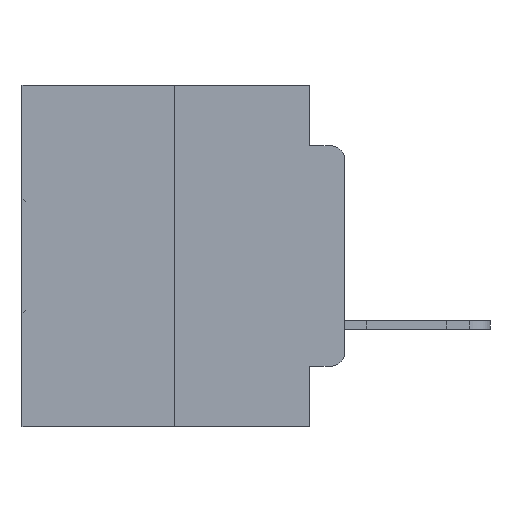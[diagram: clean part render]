
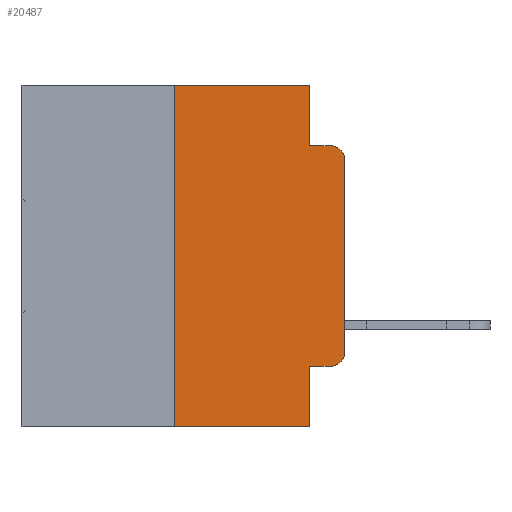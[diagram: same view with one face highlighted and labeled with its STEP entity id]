
A CAD part, left-side view. The second image highlights one B-rep face of the part: STEP entity #20487.
In plain terms, the highlighted planar face has unit normal (-1, 0, 0).
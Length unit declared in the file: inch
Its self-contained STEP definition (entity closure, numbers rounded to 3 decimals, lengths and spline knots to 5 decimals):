
#351 = VERTEX_POINT ( 'NONE', #5913 ) ;
#405 = VECTOR ( 'NONE', #18775, 39.37008 ) ;
#1139 = ORIENTED_EDGE ( 'NONE', *, *, #13608, .T. ) ;
#1945 = FACE_OUTER_BOUND ( 'NONE', #10490, .T. ) ;
#2028 = VECTOR ( 'NONE', #28562, 39.37008 ) ;
#2486 = LINE ( 'NONE', #10339, #12302 ) ;
#2933 = VERTEX_POINT ( 'NONE', #3479 ) ;
#3251 = VERTEX_POINT ( 'NONE', #19791 ) ;
#3339 = VECTOR ( 'NONE', #30224, 39.37008 ) ;
#3390 = VECTOR ( 'NONE', #20438, 39.37008 ) ;
#3479 = CARTESIAN_POINT ( 'NONE',  ( 0., 0.02, -0.0885 ) ) ;
#4576 = CARTESIAN_POINT ( 'NONE',  ( 0., 0., -0.3915 ) ) ;
#4650 = VERTEX_POINT ( 'NONE', #11251 ) ;
#5029 = DIRECTION ( 'NONE',  ( 1., 0., 0. ) ) ;
#5317 = AXIS2_PLACEMENT_3D ( 'NONE', #16862, #5029, #24354 ) ;
#5726 = ORIENTED_EDGE ( 'NONE', *, *, #31351, .T. ) ;
#5913 = CARTESIAN_POINT ( 'NONE',  ( 0., 0.25, -0.5 ) ) ;
#6045 = CARTESIAN_POINT ( 'NONE',  ( 0., 0.02, -0.1085 ) ) ;
#6817 = VECTOR ( 'NONE', #27521, 39.37008 ) ;
#6858 = CARTESIAN_POINT ( 'NONE',  ( 0., 0.051, -0.4115 ) ) ;
#6984 = DIRECTION ( 'NONE',  ( 0., 0., -1. ) ) ;
#7262 = CIRCLE ( 'NONE', #25867, 0.02 ) ;
#7264 = PLANE ( 'NONE',  #5317 ) ;
#8632 = CARTESIAN_POINT ( 'NONE',  ( 0., 0.473, 0. ) ) ;
#8911 = VECTOR ( 'NONE', #29484, 39.37008 ) ;
#9176 = ORIENTED_EDGE ( 'NONE', *, *, #18207, .F. ) ;
#9423 = CARTESIAN_POINT ( 'NONE',  ( 0., 0.051, 0. ) ) ;
#9775 = LINE ( 'NONE', #11331, #3339 ) ;
#9825 = LINE ( 'NONE', #27527, #3390 ) ;
#10070 = EDGE_CURVE ( 'NONE', #3251, #2933, #11827, .T. ) ;
#10143 = DIRECTION ( 'NONE',  ( 0., 0., -1. ) ) ;
#10339 = CARTESIAN_POINT ( 'NONE',  ( 0., 0.473, -0.5 ) ) ;
#10490 = EDGE_LOOP ( 'NONE', ( #5726, #25761, #30400, #30440, #9176, #28096, #1139, #11861, #22275, #29266 ) ) ;
#10564 = DIRECTION ( 'NONE',  ( 0., -1., 0. ) ) ;
#11251 = CARTESIAN_POINT ( 'NONE',  ( 0., 0.02, -0.4115 ) ) ;
#11331 = CARTESIAN_POINT ( 'NONE',  ( 0., 0.051, 0. ) ) ;
#11447 = EDGE_CURVE ( 'NONE', #21841, #3251, #9775, .T. ) ;
#11827 = LINE ( 'NONE', #21845, #405 ) ;
#11861 = ORIENTED_EDGE ( 'NONE', *, *, #20864, .F. ) ;
#12302 = VECTOR ( 'NONE', #10564, 39.37008 ) ;
#12610 = CARTESIAN_POINT ( 'NONE',  ( 0., 0.25, 0. ) ) ;
#12850 = CARTESIAN_POINT ( 'NONE',  ( 0., 0., 0. ) ) ;
#12901 = EDGE_CURVE ( 'NONE', #24994, #4650, #30842, .T. ) ;
#13608 = EDGE_CURVE ( 'NONE', #351, #26804, #2486, .T. ) ;
#13958 = DIRECTION ( 'NONE',  ( -1., 0., 0. ) ) ;
#15592 = DIRECTION ( 'NONE',  ( 0., 0., 1. ) ) ;
#16032 = VERTEX_POINT ( 'NONE', #23513 ) ;
#16079 = VERTEX_POINT ( 'NONE', #23188 ) ;
#16862 = CARTESIAN_POINT ( 'NONE',  ( 0., 0.473, 0. ) ) ;
#17411 = DIRECTION ( 'NONE',  ( -1., 0., 0. ) ) ;
#17823 = EDGE_CURVE ( 'NONE', #16032, #2933, #18289, .T. ) ;
#18207 = EDGE_CURVE ( 'NONE', #16079, #21841, #29977, .T. ) ;
#18289 = CIRCLE ( 'NONE', #25329, 0.02 ) ;
#18775 = DIRECTION ( 'NONE',  ( 0., -1., 0. ) ) ;
#19086 = VECTOR ( 'NONE', #15592, 39.37008 ) ;
#19791 = CARTESIAN_POINT ( 'NONE',  ( 0., 0.051, -0.0885 ) ) ;
#20438 = DIRECTION ( 'NONE',  ( 0., 0., -1. ) ) ;
#20487 = ADVANCED_FACE ( 'NONE', ( #1945 ), #7264, .F. ) ;
#20864 = EDGE_CURVE ( 'NONE', #24994, #26804, #9825, .T. ) ;
#21079 = VERTEX_POINT ( 'NONE', #4576 ) ;
#21841 = VERTEX_POINT ( 'NONE', #9423 ) ;
#21845 = CARTESIAN_POINT ( 'NONE',  ( 0., 0.051, -0.0885 ) ) ;
#22078 = CARTESIAN_POINT ( 'NONE',  ( 0., 0.051, -0.4115 ) ) ;
#22257 = CARTESIAN_POINT ( 'NONE',  ( 0., 0.02, -0.3915 ) ) ;
#22275 = ORIENTED_EDGE ( 'NONE', *, *, #12901, .T. ) ;
#22459 = LINE ( 'NONE', #12850, #19086 ) ;
#23188 = CARTESIAN_POINT ( 'NONE',  ( 0., 0.25, 0. ) ) ;
#23513 = CARTESIAN_POINT ( 'NONE',  ( 0., 0., -0.1085 ) ) ;
#24354 = DIRECTION ( 'NONE',  ( 0., 0., -1. ) ) ;
#24994 = VERTEX_POINT ( 'NONE', #6858 ) ;
#25329 = AXIS2_PLACEMENT_3D ( 'NONE', #6045, #13958, #6984 ) ;
#25761 = ORIENTED_EDGE ( 'NONE', *, *, #17823, .T. ) ;
#25867 = AXIS2_PLACEMENT_3D ( 'NONE', #22257, #17411, #10143 ) ;
#26454 = EDGE_CURVE ( 'NONE', #4650, #21079, #7262, .T. ) ;
#26804 = VERTEX_POINT ( 'NONE', #28732 ) ;
#27521 = DIRECTION ( 'NONE',  ( 0., 0., 1. ) ) ;
#27527 = CARTESIAN_POINT ( 'NONE',  ( 0., 0.051, 0. ) ) ;
#27682 = EDGE_CURVE ( 'NONE', #351, #16079, #29821, .T. ) ;
#28096 = ORIENTED_EDGE ( 'NONE', *, *, #27682, .F. ) ;
#28562 = DIRECTION ( 'NONE',  ( 0., -1., 0. ) ) ;
#28732 = CARTESIAN_POINT ( 'NONE',  ( 0., 0.051, -0.5 ) ) ;
#29266 = ORIENTED_EDGE ( 'NONE', *, *, #26454, .T. ) ;
#29484 = DIRECTION ( 'NONE',  ( 0., -1., 0. ) ) ;
#29821 = LINE ( 'NONE', #12610, #6817 ) ;
#29977 = LINE ( 'NONE', #8632, #2028 ) ;
#30224 = DIRECTION ( 'NONE',  ( 0., 0., -1. ) ) ;
#30400 = ORIENTED_EDGE ( 'NONE', *, *, #10070, .F. ) ;
#30440 = ORIENTED_EDGE ( 'NONE', *, *, #11447, .F. ) ;
#30842 = LINE ( 'NONE', #22078, #8911 ) ;
#31351 = EDGE_CURVE ( 'NONE', #21079, #16032, #22459, .T. ) ;
